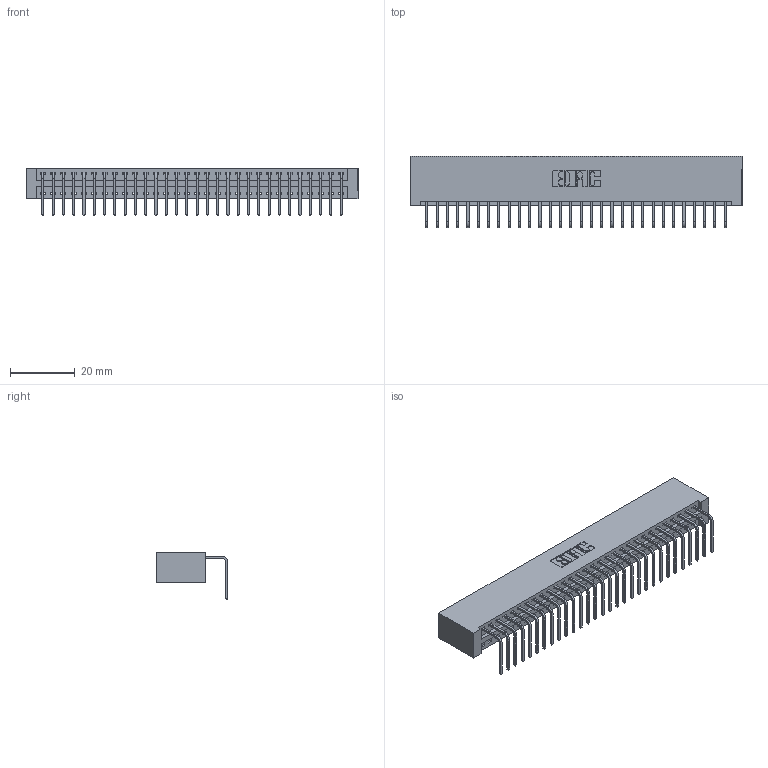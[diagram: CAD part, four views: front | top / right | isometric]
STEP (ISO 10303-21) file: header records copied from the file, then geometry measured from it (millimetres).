
FILE_DESCRIPTION (( 'STEP AP203' ), '1' );
FILE_NAME ('396-030-558-101.STEP', '2018-09-05T07:43:33', ( '' ), ( '' ), 'SwSTEP 2.0', 'SolidWorks 2016', '' );
FILE_SCHEMA (( 'CONFIG_CONTROL_DESIGN' ));
Length unit declared in the file: inch
Products named in the file (3): 345-292-001_558 Tail - 2; 396-030-558-101; 346 Part_No Mounting Lugs
Assembly tree (31 placements, depth 2):
  396-030-558-101
    346 Part_No Mounting Lugs
    345-292-001_558 Tail - 2  x30
Bounding box: 102.49 x 22.16 x 14.73 mm (x, y, z)
Volume: 10377.1 mm3; surface area: 13512 mm2
Topology: 31 solids, 31 shells, 1914 faces, 5765 edges, 3802 vertices
Faces by surface type: plane 1332, cylinder 582
Entity records: 20041 total; most frequent: CARTESIAN_POINT 3446, ORIENTED_EDGE 3410, DIRECTION 3049, EDGE_CURVE 1705, LINE 1461, VECTOR 1461, VERTEX_POINT 1134, AXIS2_PLACEMENT_3D 794
